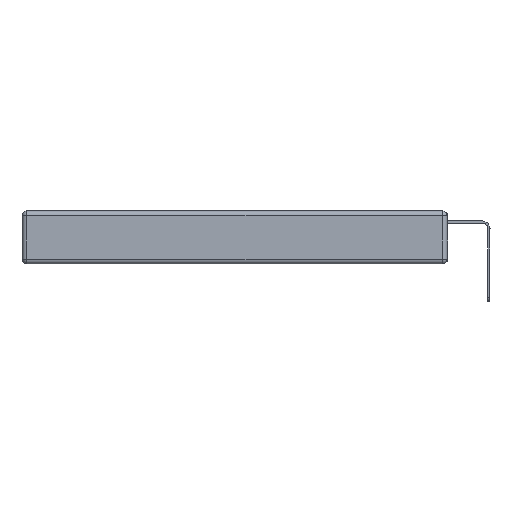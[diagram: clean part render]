
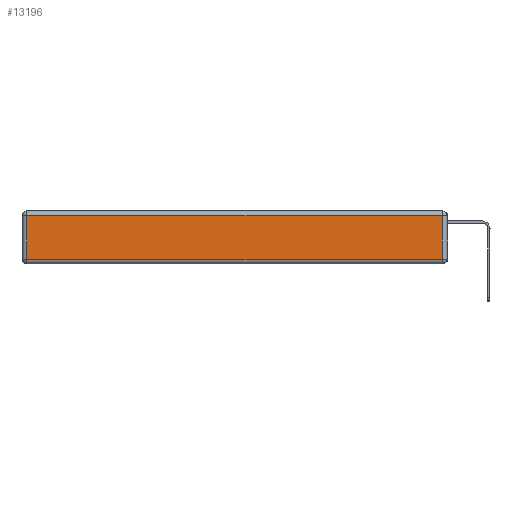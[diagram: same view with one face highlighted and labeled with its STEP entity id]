
A CAD part, left-side view. The second image highlights one B-rep face of the part: STEP entity #13196.
In plain terms, the highlighted planar face has unit normal (-1, 0, 0).
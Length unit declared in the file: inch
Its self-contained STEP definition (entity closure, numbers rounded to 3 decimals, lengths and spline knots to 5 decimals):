
#348 = DIRECTION ( 'NONE',  ( 0., -1., 0. ) ) ;
#1322 = LINE ( 'NONE', #6658, #13757 ) ;
#1575 = CARTESIAN_POINT ( 'NONE',  ( 0., 0., -0.313 ) ) ;
#1787 = LINE ( 'NONE', #1575, #4187 ) ;
#2041 = CARTESIAN_POINT ( 'NONE',  ( 0., 2.72, -0.313 ) ) ;
#2231 = CARTESIAN_POINT ( 'NONE',  ( 0., 2.72, -0.03 ) ) ;
#2514 = VERTEX_POINT ( 'NONE', #2231 ) ;
#2831 = EDGE_LOOP ( 'NONE', ( #4204, #14511, #13081, #6011 ) ) ;
#3329 = VERTEX_POINT ( 'NONE', #2041 ) ;
#3636 = DIRECTION ( 'NONE',  ( 0., 0., 1. ) ) ;
#4187 = VECTOR ( 'NONE', #348, 39.37008 ) ;
#4204 = ORIENTED_EDGE ( 'NONE', *, *, #5283, .T. ) ;
#4331 = VECTOR ( 'NONE', #9623, 39.37008 ) ;
#4547 = AXIS2_PLACEMENT_3D ( 'NONE', #10735, #12042, #3636 ) ;
#4987 = EDGE_CURVE ( 'NONE', #9223, #2514, #14416, .T. ) ;
#5283 = EDGE_CURVE ( 'NONE', #3329, #12829, #1787, .T. ) ;
#5741 = CARTESIAN_POINT ( 'NONE',  ( 0., 2.75, -0.03 ) ) ;
#6011 = ORIENTED_EDGE ( 'NONE', *, *, #9284, .T. ) ;
#6154 = LINE ( 'NONE', #6175, #4331 ) ;
#6175 = CARTESIAN_POINT ( 'NONE',  ( 0., 2.72, -0.343 ) ) ;
#6658 = CARTESIAN_POINT ( 'NONE',  ( 0., 0.03, -0.343 ) ) ;
#9223 = VERTEX_POINT ( 'NONE', #13968 ) ;
#9284 = EDGE_CURVE ( 'NONE', #2514, #3329, #6154, .T. ) ;
#9623 = DIRECTION ( 'NONE',  ( 0., 0., -1. ) ) ;
#10603 = DIRECTION ( 'NONE',  ( 0., 1., 0. ) ) ;
#10735 = CARTESIAN_POINT ( 'NONE',  ( 0., 0., -0.343 ) ) ;
#10812 = EDGE_CURVE ( 'NONE', #12829, #9223, #1322, .T. ) ;
#11112 = CARTESIAN_POINT ( 'NONE',  ( 0., 0.03, -0.313 ) ) ;
#11275 = FACE_OUTER_BOUND ( 'NONE', #2831, .T. ) ;
#12042 = DIRECTION ( 'NONE',  ( -1., 0., 0. ) ) ;
#12662 = DIRECTION ( 'NONE',  ( 0., 0., 1. ) ) ;
#12829 = VERTEX_POINT ( 'NONE', #11112 ) ;
#13081 = ORIENTED_EDGE ( 'NONE', *, *, #4987, .T. ) ;
#13131 = PLANE ( 'NONE',  #4547 ) ;
#13196 = ADVANCED_FACE ( 'NONE', ( #11275 ), #13131, .T. ) ;
#13757 = VECTOR ( 'NONE', #12662, 39.37008 ) ;
#13968 = CARTESIAN_POINT ( 'NONE',  ( 0., 0.03, -0.03 ) ) ;
#14416 = LINE ( 'NONE', #5741, #14798 ) ;
#14511 = ORIENTED_EDGE ( 'NONE', *, *, #10812, .T. ) ;
#14798 = VECTOR ( 'NONE', #10603, 39.37008 ) ;
